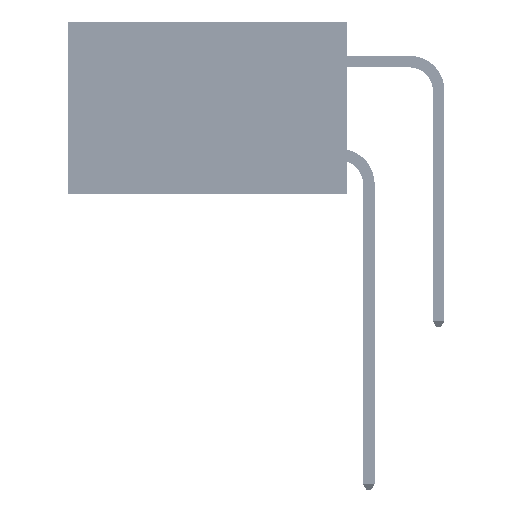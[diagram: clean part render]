
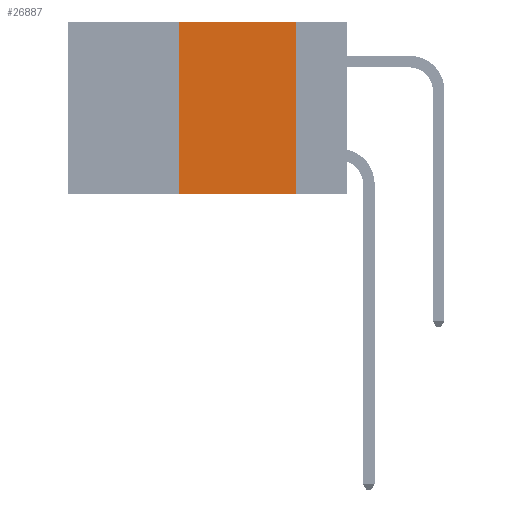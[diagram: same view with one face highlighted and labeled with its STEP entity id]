
A CAD part, left-side view. The second image highlights one B-rep face of the part: STEP entity #26887.
In plain terms, the highlighted planar face has unit normal (-1, 0, 0).
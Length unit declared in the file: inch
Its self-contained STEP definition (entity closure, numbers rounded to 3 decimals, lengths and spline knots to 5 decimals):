
#2762 = LINE ( 'NONE', #48861, #8370 ) ;
#3062 = CARTESIAN_POINT ( 'NONE',  ( 0., 0.11, -0.37 ) ) ;
#4370 = CARTESIAN_POINT ( 'NONE',  ( 0., 0.11, 0. ) ) ;
#7222 = CARTESIAN_POINT ( 'NONE',  ( 0., 0.11, 0. ) ) ;
#7922 = LINE ( 'NONE', #34465, #37772 ) ;
#8370 = VECTOR ( 'NONE', #48614, 39.37008 ) ;
#8852 = DIRECTION ( 'NONE',  ( 0., 0., -1. ) ) ;
#9091 = FACE_OUTER_BOUND ( 'NONE', #15336, .T. ) ;
#9459 = ORIENTED_EDGE ( 'NONE', *, *, #14361, .F. ) ;
#12975 = VERTEX_POINT ( 'NONE', #16315 ) ;
#14361 = EDGE_CURVE ( 'NONE', #28613, #38781, #2762, .T. ) ;
#14912 = EDGE_CURVE ( 'NONE', #38781, #29624, #44803, .T. ) ;
#15336 = EDGE_LOOP ( 'NONE', ( #18267, #9459, #21724, #37470 ) ) ;
#16195 = AXIS2_PLACEMENT_3D ( 'NONE', #47663, #39651, #8852 ) ;
#16315 = CARTESIAN_POINT ( 'NONE',  ( 0., 0.36, -0.37 ) ) ;
#17715 = CARTESIAN_POINT ( 'NONE',  ( 0., 0.36, 0. ) ) ;
#18267 = ORIENTED_EDGE ( 'NONE', *, *, #14912, .F. ) ;
#18289 = EDGE_CURVE ( 'NONE', #12975, #28613, #42015, .T. ) ;
#20370 = PLANE ( 'NONE',  #16195 ) ;
#21724 = ORIENTED_EDGE ( 'NONE', *, *, #18289, .F. ) ;
#22987 = DIRECTION ( 'NONE',  ( 0., 0., 1. ) ) ;
#26887 = ADVANCED_FACE ( 'NONE', ( #9091 ), #20370, .F. ) ;
#28613 = VERTEX_POINT ( 'NONE', #17715 ) ;
#29624 = VERTEX_POINT ( 'NONE', #3062 ) ;
#31585 = VECTOR ( 'NONE', #41042, 39.37008 ) ;
#34465 = CARTESIAN_POINT ( 'NONE',  ( 0., 0.6, -0.37 ) ) ;
#34993 = CARTESIAN_POINT ( 'NONE',  ( 0., 0.36, 0. ) ) ;
#37470 = ORIENTED_EDGE ( 'NONE', *, *, #44434, .T. ) ;
#37735 = DIRECTION ( 'NONE',  ( 0., -1., 0. ) ) ;
#37772 = VECTOR ( 'NONE', #37735, 39.37008 ) ;
#38781 = VERTEX_POINT ( 'NONE', #4370 ) ;
#39651 = DIRECTION ( 'NONE',  ( 1., 0., 0. ) ) ;
#39721 = VECTOR ( 'NONE', #22987, 39.37008 ) ;
#41042 = DIRECTION ( 'NONE',  ( 0., 0., -1. ) ) ;
#42015 = LINE ( 'NONE', #34993, #39721 ) ;
#44434 = EDGE_CURVE ( 'NONE', #12975, #29624, #7922, .T. ) ;
#44803 = LINE ( 'NONE', #7222, #31585 ) ;
#47663 = CARTESIAN_POINT ( 'NONE',  ( 0., 0.6, 0. ) ) ;
#48614 = DIRECTION ( 'NONE',  ( 0., -1., 0. ) ) ;
#48861 = CARTESIAN_POINT ( 'NONE',  ( 0., 0.6, 0. ) ) ;
